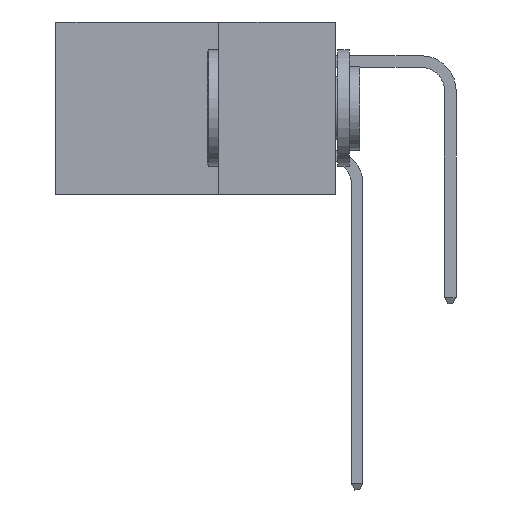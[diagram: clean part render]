
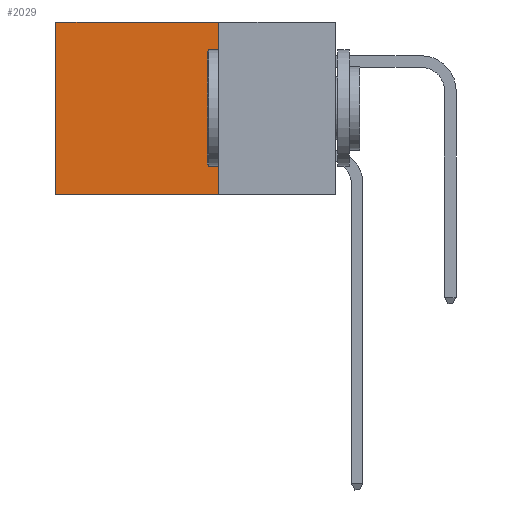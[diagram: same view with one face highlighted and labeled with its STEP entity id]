
A CAD part, left-side view. The second image highlights one B-rep face of the part: STEP entity #2029.
In plain terms, the highlighted planar face has unit normal (-1, 0, 0).
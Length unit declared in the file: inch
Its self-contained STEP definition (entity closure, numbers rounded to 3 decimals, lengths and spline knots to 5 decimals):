
#2029 = ADVANCED_FACE ( 'NONE', ( #21748 ), #19801, .F. ) ;
#3173 = EDGE_CURVE ( 'NONE', #12515, #14175, #21978, .T. ) ;
#3222 = CARTESIAN_POINT ( 'NONE',  ( 0.2875, 0.25, -0.37 ) ) ;
#6058 = CARTESIAN_POINT ( 'NONE',  ( 0.2875, 0.6, 0. ) ) ;
#7098 = VECTOR ( 'NONE', #14286, 39.37008 ) ;
#7139 = VERTEX_POINT ( 'NONE', #13755 ) ;
#7146 = ORIENTED_EDGE ( 'NONE', *, *, #12344, .T. ) ;
#8392 = CARTESIAN_POINT ( 'NONE',  ( 0.2875, 0.25, 0. ) ) ;
#8819 = LINE ( 'NONE', #8392, #18742 ) ;
#8890 = VECTOR ( 'NONE', #9984, 39.37008 ) ;
#9984 = DIRECTION ( 'NONE',  ( 0., 1., 0. ) ) ;
#12061 = DIRECTION ( 'NONE',  ( 0., 0., -1. ) ) ;
#12344 = EDGE_CURVE ( 'NONE', #7139, #18135, #23768, .T. ) ;
#12515 = VERTEX_POINT ( 'NONE', #14524 ) ;
#12966 = CARTESIAN_POINT ( 'NONE',  ( 0.2875, 0.6, 0. ) ) ;
#13271 = EDGE_CURVE ( 'NONE', #18135, #14175, #22007, .T. ) ;
#13652 = EDGE_CURVE ( 'NONE', #7139, #12515, #8819, .T. ) ;
#13755 = CARTESIAN_POINT ( 'NONE',  ( 0.2875, 0.25, 0. ) ) ;
#14175 = VERTEX_POINT ( 'NONE', #17741 ) ;
#14286 = DIRECTION ( 'NONE',  ( 0., 1., 0. ) ) ;
#14461 = ORIENTED_EDGE ( 'NONE', *, *, #3173, .F. ) ;
#14524 = CARTESIAN_POINT ( 'NONE',  ( 0.2875, 0.25, -0.37 ) ) ;
#16540 = ORIENTED_EDGE ( 'NONE', *, *, #13652, .F. ) ;
#16571 = ORIENTED_EDGE ( 'NONE', *, *, #13271, .T. ) ;
#17741 = CARTESIAN_POINT ( 'NONE',  ( 0.2875, 0.6, -0.37 ) ) ;
#18135 = VERTEX_POINT ( 'NONE', #6058 ) ;
#18326 = DIRECTION ( 'NONE',  ( 0., 0., -1. ) ) ;
#18336 = DIRECTION ( 'NONE',  ( 1., 0., 0. ) ) ;
#18742 = VECTOR ( 'NONE', #12061, 39.37008 ) ;
#18754 = EDGE_LOOP ( 'NONE', ( #16571, #14461, #16540, #7146 ) ) ;
#19353 = CARTESIAN_POINT ( 'NONE',  ( 0.2875, 0.25, 0. ) ) ;
#19801 = PLANE ( 'NONE',  #24089 ) ;
#21434 = VECTOR ( 'NONE', #22303, 39.37008 ) ;
#21748 = FACE_OUTER_BOUND ( 'NONE', #18754, .T. ) ;
#21978 = LINE ( 'NONE', #3222, #7098 ) ;
#22007 = LINE ( 'NONE', #12966, #21434 ) ;
#22303 = DIRECTION ( 'NONE',  ( 0., 0., -1. ) ) ;
#22981 = CARTESIAN_POINT ( 'NONE',  ( 0.2875, 0.25, 0. ) ) ;
#23768 = LINE ( 'NONE', #22981, #8890 ) ;
#24089 = AXIS2_PLACEMENT_3D ( 'NONE', #19353, #18336, #18326 ) ;
